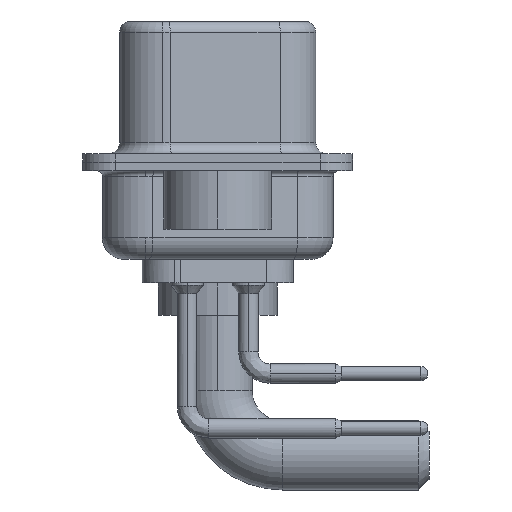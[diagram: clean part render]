
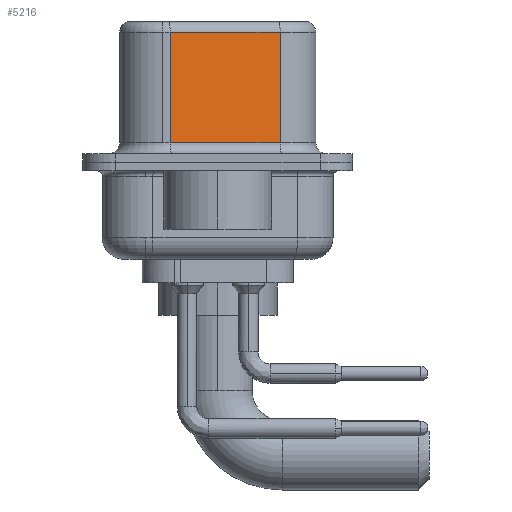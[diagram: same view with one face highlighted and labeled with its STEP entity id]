
A CAD part, left-side view. The second image highlights one B-rep face of the part: STEP entity #5216.
In plain terms, the highlighted planar face has unit normal (-0.985, -0.174, 0).
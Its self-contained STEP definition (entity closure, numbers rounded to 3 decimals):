
#1427 = VERTEX_POINT ( 'NONE', #9350 ) ;
#2640 = DIRECTION ( 'NONE',  ( 0.985, 0.174, 0. ) ) ;
#2940 = CARTESIAN_POINT ( 'NONE',  ( 4.58, -2.897, 6.02 ) ) ;
#3031 = LINE ( 'NONE', #8998, #14668 ) ;
#3117 = EDGE_CURVE ( 'NONE', #1427, #15933, #12277, .T. ) ;
#3741 = AXIS2_PLACEMENT_3D ( 'NONE', #16158, #2640, #5488 ) ;
#4795 = EDGE_CURVE ( 'NONE', #13527, #15354, #3031, .T. ) ;
#4840 = DIRECTION ( 'NONE',  ( 0., 0., -1. ) ) ;
#4880 = ORIENTED_EDGE ( 'NONE', *, *, #4795, .F. ) ;
#5216 = ADVANCED_FACE ( 'NONE', ( #11546 ), #17640, .F. ) ;
#5488 = DIRECTION ( 'NONE',  ( -0.174, 0.985, 0. ) ) ;
#6076 = DIRECTION ( 'NONE',  ( 0., 0., -1. ) ) ;
#6573 = LINE ( 'NONE', #16685, #17304 ) ;
#6697 = ORIENTED_EDGE ( 'NONE', *, *, #3117, .T. ) ;
#8421 = CARTESIAN_POINT ( 'NONE',  ( 4.58, -2.897, 0.9 ) ) ;
#8621 = EDGE_CURVE ( 'NONE', #13527, #1427, #13513, .T. ) ;
#8998 = CARTESIAN_POINT ( 'NONE',  ( 4.58, -2.897, 6.52 ) ) ;
#9350 = CARTESIAN_POINT ( 'NONE',  ( 3.68, 2.203, 6.02 ) ) ;
#9894 = CARTESIAN_POINT ( 'NONE',  ( 4.58, -2.897, 6.02 ) ) ;
#10375 = DIRECTION ( 'NONE',  ( -0.174, 0.985, 0. ) ) ;
#11546 = FACE_OUTER_BOUND ( 'NONE', #15648, .T. ) ;
#12277 = LINE ( 'NONE', #18274, #16491 ) ;
#12555 = DIRECTION ( 'NONE',  ( 0.174, -0.985, 0. ) ) ;
#13310 = ORIENTED_EDGE ( 'NONE', *, *, #15236, .T. ) ;
#13513 = LINE ( 'NONE', #2940, #15384 ) ;
#13527 = VERTEX_POINT ( 'NONE', #9894 ) ;
#14668 = VECTOR ( 'NONE', #6076, 1000. ) ;
#14752 = ORIENTED_EDGE ( 'NONE', *, *, #8621, .T. ) ;
#14801 = CARTESIAN_POINT ( 'NONE',  ( 3.68, 2.203, 0.9 ) ) ;
#15236 = EDGE_CURVE ( 'NONE', #15933, #15354, #6573, .T. ) ;
#15354 = VERTEX_POINT ( 'NONE', #8421 ) ;
#15384 = VECTOR ( 'NONE', #10375, 1000. ) ;
#15648 = EDGE_LOOP ( 'NONE', ( #4880, #14752, #6697, #13310 ) ) ;
#15933 = VERTEX_POINT ( 'NONE', #14801 ) ;
#16158 = CARTESIAN_POINT ( 'NONE',  ( 4.58, -2.897, 6.52 ) ) ;
#16491 = VECTOR ( 'NONE', #4840, 1000. ) ;
#16685 = CARTESIAN_POINT ( 'NONE',  ( 4.58, -2.897, 0.9 ) ) ;
#17304 = VECTOR ( 'NONE', #12555, 1000. ) ;
#17640 = PLANE ( 'NONE',  #3741 ) ;
#18274 = CARTESIAN_POINT ( 'NONE',  ( 3.68, 2.203, 6.52 ) ) ;
